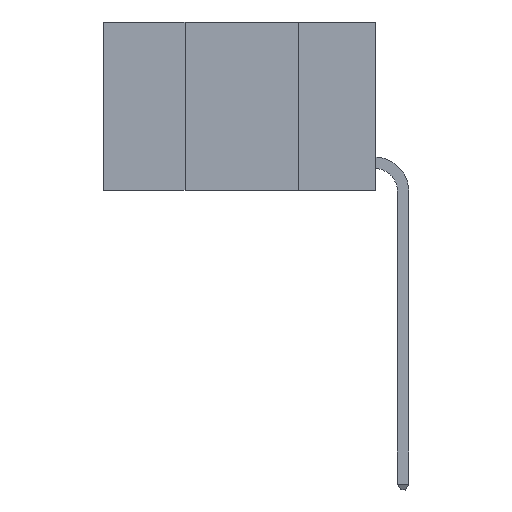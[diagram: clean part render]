
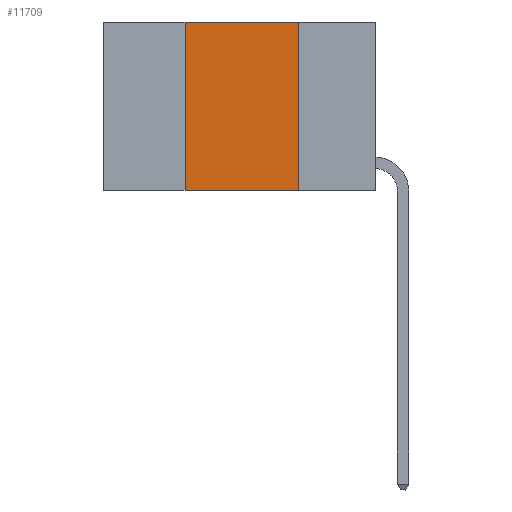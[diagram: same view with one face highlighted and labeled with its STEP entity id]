
A CAD part, left-side view. The second image highlights one B-rep face of the part: STEP entity #11709.
In plain terms, the highlighted planar face has unit normal (-1, 0, 0).
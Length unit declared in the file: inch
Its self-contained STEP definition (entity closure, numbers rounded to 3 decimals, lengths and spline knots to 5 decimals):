
#304 = VERTEX_POINT ( 'NONE', #8578 ) ;
#456 = DIRECTION ( 'NONE',  ( 0., 0., -1. ) ) ;
#505 = CARTESIAN_POINT ( 'NONE',  ( 0., 0.42, 0. ) ) ;
#849 = LINE ( 'NONE', #2078, #10204 ) ;
#1061 = LINE ( 'NONE', #4735, #7635 ) ;
#1733 = DIRECTION ( 'NONE',  ( 0., 0., 1. ) ) ;
#2078 = CARTESIAN_POINT ( 'NONE',  ( 0., 0.17, 0. ) ) ;
#3090 = LINE ( 'NONE', #505, #15193 ) ;
#3383 = VERTEX_POINT ( 'NONE', #5158 ) ;
#4006 = VERTEX_POINT ( 'NONE', #8802 ) ;
#4421 = ORIENTED_EDGE ( 'NONE', *, *, #6110, .F. ) ;
#4735 = CARTESIAN_POINT ( 'NONE',  ( 0., 0.6, -0.37 ) ) ;
#5158 = CARTESIAN_POINT ( 'NONE',  ( 0., 0.42, 0. ) ) ;
#5358 = EDGE_CURVE ( 'NONE', #4006, #14515, #1061, .T. ) ;
#5366 = CARTESIAN_POINT ( 'NONE',  ( 0., 0.6, 0. ) ) ;
#6110 = EDGE_CURVE ( 'NONE', #3383, #304, #12569, .T. ) ;
#6160 = EDGE_CURVE ( 'NONE', #4006, #3383, #3090, .T. ) ;
#6583 = ORIENTED_EDGE ( 'NONE', *, *, #8614, .F. ) ;
#6601 = PLANE ( 'NONE',  #13188 ) ;
#6940 = FACE_OUTER_BOUND ( 'NONE', #11733, .T. ) ;
#7635 = VECTOR ( 'NONE', #12996, 39.37008 ) ;
#7815 = DIRECTION ( 'NONE',  ( 1., 0., 0. ) ) ;
#7926 = ORIENTED_EDGE ( 'NONE', *, *, #5358, .T. ) ;
#8578 = CARTESIAN_POINT ( 'NONE',  ( 0., 0.17, 0. ) ) ;
#8614 = EDGE_CURVE ( 'NONE', #304, #14515, #849, .T. ) ;
#8802 = CARTESIAN_POINT ( 'NONE',  ( 0., 0.42, -0.37 ) ) ;
#9545 = VECTOR ( 'NONE', #10157, 39.37008 ) ;
#9821 = CARTESIAN_POINT ( 'NONE',  ( 0., 0.17, -0.37 ) ) ;
#10157 = DIRECTION ( 'NONE',  ( 0., -1., 0. ) ) ;
#10204 = VECTOR ( 'NONE', #15015, 39.37008 ) ;
#11709 = ADVANCED_FACE ( 'NONE', ( #6940 ), #6601, .F. ) ;
#11733 = EDGE_LOOP ( 'NONE', ( #6583, #4421, #15249, #7926 ) ) ;
#12374 = CARTESIAN_POINT ( 'NONE',  ( 0., 0.6, 0. ) ) ;
#12569 = LINE ( 'NONE', #12374, #9545 ) ;
#12996 = DIRECTION ( 'NONE',  ( 0., -1., 0. ) ) ;
#13188 = AXIS2_PLACEMENT_3D ( 'NONE', #5366, #7815, #456 ) ;
#14515 = VERTEX_POINT ( 'NONE', #9821 ) ;
#15015 = DIRECTION ( 'NONE',  ( 0., 0., -1. ) ) ;
#15193 = VECTOR ( 'NONE', #1733, 39.37008 ) ;
#15249 = ORIENTED_EDGE ( 'NONE', *, *, #6160, .F. ) ;
